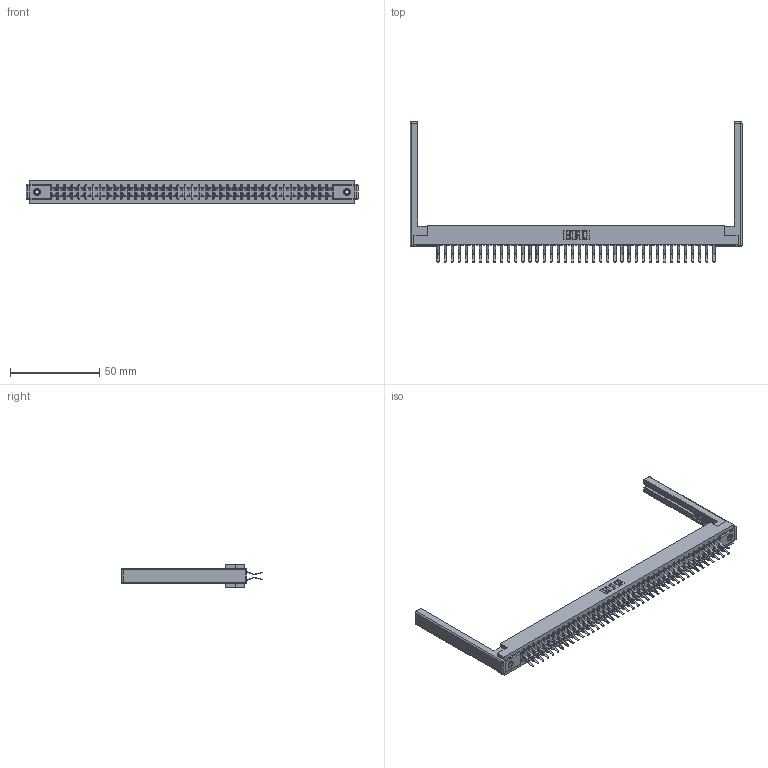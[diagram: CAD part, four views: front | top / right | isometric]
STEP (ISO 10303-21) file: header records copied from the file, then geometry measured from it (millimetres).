
FILE_DESCRIPTION (( 'STEP AP203' ), '1' );
FILE_NAME ('357-080-560-268.STEP', '2019-09-19T16:17:01', ( '' ), ( '' ), 'SwSTEP 2.0', 'SolidWorks 2016', '' );
FILE_SCHEMA (( 'CONFIG_CONTROL_DESIGN' ));
Length unit declared in the file: inch
Products named in the file (5): 307-220-068; 307 Part_.156 Dia Mounting Holes; 357-080-560-268; 307-290-001_560; 345-250-001_345-250-001-102
Assembly tree (85 placements, depth 2):
  357-080-560-268
    307 Part_.156 Dia Mounting Holes
    307-290-001_560  x80
    307-220-068  x2
    345-250-001_345-250-001-102  x2
Bounding box: 185.93 x 78.69 x 12.7 mm (x, y, z)
Volume: 24237.4 mm3; surface area: 28774.4 mm2
Topology: 85 solids, 85 shells, 4313 faces, 12073 edges, 7810 vertices
Faces by surface type: plane 2798, cylinder 1409, sphere 90, cone 12, torus 4
Entity records: 38681 total; most frequent: CARTESIAN_POINT 6305, ORIENTED_EDGE 6240, DIRECTION 6192, EDGE_CURVE 3120, VECTOR 2390, LINE 2390, VERTEX_POINT 2014, AXIS2_PLACEMENT_3D 1901
